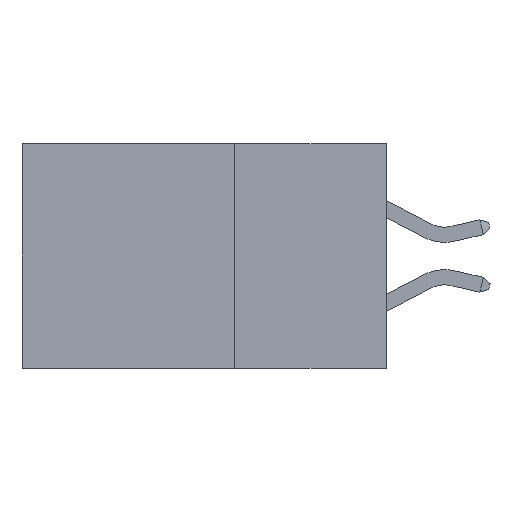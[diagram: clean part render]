
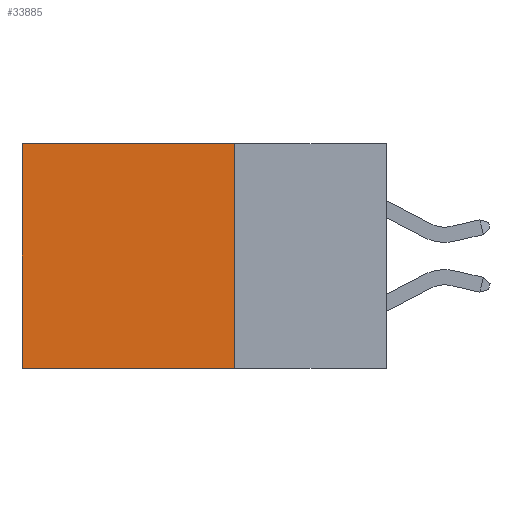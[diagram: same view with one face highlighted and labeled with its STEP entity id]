
A CAD part, left-side view. The second image highlights one B-rep face of the part: STEP entity #33885.
In plain terms, the highlighted planar face has unit normal (-1, 0, 0).
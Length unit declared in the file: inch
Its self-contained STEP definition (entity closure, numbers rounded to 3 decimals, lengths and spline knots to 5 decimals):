
#209 = CARTESIAN_POINT ( 'NONE',  ( 0.298, 0.6, -0.37 ) ) ;
#1078 = ORIENTED_EDGE ( 'NONE', *, *, #6612, .T. ) ;
#1789 = ORIENTED_EDGE ( 'NONE', *, *, #18305, .F. ) ;
#4161 = VECTOR ( 'NONE', #5288, 39.37008 ) ;
#4688 = CARTESIAN_POINT ( 'NONE',  ( 0.298, 0.25, -0.37 ) ) ;
#5288 = DIRECTION ( 'NONE',  ( 0., 0., -1. ) ) ;
#6328 = EDGE_LOOP ( 'NONE', ( #1078, #1789, #17089, #14305 ) ) ;
#6612 = EDGE_CURVE ( 'NONE', #16506, #10015, #11786, .T. ) ;
#7350 = CARTESIAN_POINT ( 'NONE',  ( 0.298, 0.6, 0. ) ) ;
#8302 = AXIS2_PLACEMENT_3D ( 'NONE', #18347, #10631, #10860 ) ;
#10015 = VERTEX_POINT ( 'NONE', #209 ) ;
#10285 = DIRECTION ( 'NONE',  ( 0., 1., 0. ) ) ;
#10402 = VECTOR ( 'NONE', #32410, 39.37008 ) ;
#10631 = DIRECTION ( 'NONE',  ( 1., 0., 0. ) ) ;
#10860 = DIRECTION ( 'NONE',  ( 0., 0., -1. ) ) ;
#11129 = LINE ( 'NONE', #21103, #4161 ) ;
#11419 = CARTESIAN_POINT ( 'NONE',  ( 0.298, 0.25, 0. ) ) ;
#11786 = LINE ( 'NONE', #22258, #18820 ) ;
#13418 = PLANE ( 'NONE',  #8302 ) ;
#13870 = FACE_OUTER_BOUND ( 'NONE', #6328, .T. ) ;
#14305 = ORIENTED_EDGE ( 'NONE', *, *, #14745, .T. ) ;
#14745 = EDGE_CURVE ( 'NONE', #23259, #16506, #25173, .T. ) ;
#16059 = CARTESIAN_POINT ( 'NONE',  ( 0.298, 0.25, -0.37 ) ) ;
#16506 = VERTEX_POINT ( 'NONE', #7350 ) ;
#17089 = ORIENTED_EDGE ( 'NONE', *, *, #31589, .F. ) ;
#18305 = EDGE_CURVE ( 'NONE', #24503, #10015, #22831, .T. ) ;
#18347 = CARTESIAN_POINT ( 'NONE',  ( 0.298, 0.25, 0. ) ) ;
#18820 = VECTOR ( 'NONE', #25101, 39.37008 ) ;
#21103 = CARTESIAN_POINT ( 'NONE',  ( 0.298, 0.25, 0. ) ) ;
#22258 = CARTESIAN_POINT ( 'NONE',  ( 0.298, 0.6, 0. ) ) ;
#22831 = LINE ( 'NONE', #4688, #27341 ) ;
#23259 = VERTEX_POINT ( 'NONE', #24580 ) ;
#24503 = VERTEX_POINT ( 'NONE', #16059 ) ;
#24580 = CARTESIAN_POINT ( 'NONE',  ( 0.298, 0.25, 0. ) ) ;
#25101 = DIRECTION ( 'NONE',  ( 0., 0., -1. ) ) ;
#25173 = LINE ( 'NONE', #11419, #10402 ) ;
#27341 = VECTOR ( 'NONE', #10285, 39.37008 ) ;
#31589 = EDGE_CURVE ( 'NONE', #23259, #24503, #11129, .T. ) ;
#32410 = DIRECTION ( 'NONE',  ( 0., 1., 0. ) ) ;
#33885 = ADVANCED_FACE ( 'NONE', ( #13870 ), #13418, .F. ) ;
